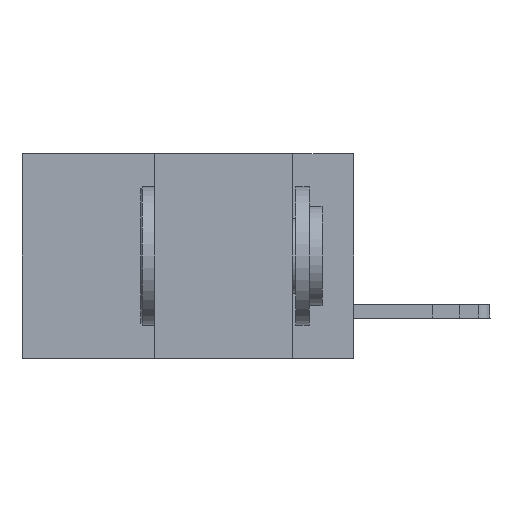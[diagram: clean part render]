
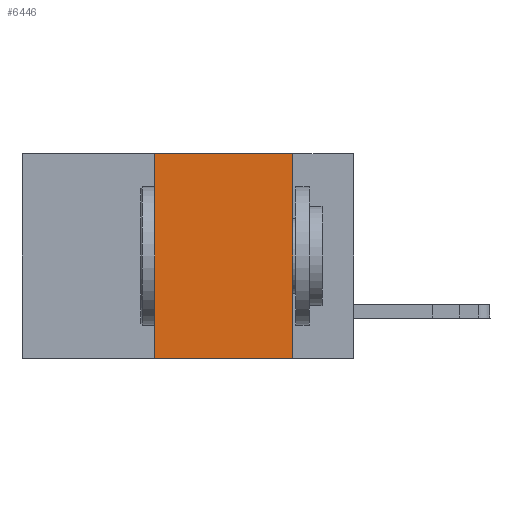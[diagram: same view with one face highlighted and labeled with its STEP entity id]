
A CAD part, left-side view. The second image highlights one B-rep face of the part: STEP entity #6446.
In plain terms, the highlighted planar face has unit normal (-1, 0, 0).
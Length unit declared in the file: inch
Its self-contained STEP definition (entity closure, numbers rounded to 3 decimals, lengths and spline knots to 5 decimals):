
#404 = LINE ( 'NONE', #10744, #22834 ) ;
#2737 = EDGE_CURVE ( 'NONE', #16615, #4697, #3067, .T. ) ;
#3067 = LINE ( 'NONE', #9073, #10866 ) ;
#4490 = PLANE ( 'NONE',  #12348 ) ;
#4584 = ORIENTED_EDGE ( 'NONE', *, *, #37653, .F. ) ;
#4697 = VERTEX_POINT ( 'NONE', #30077 ) ;
#6210 = LINE ( 'NONE', #21986, #13987 ) ;
#6305 = CARTESIAN_POINT ( 'NONE',  ( 0., 0.11, 0. ) ) ;
#6446 = ADVANCED_FACE ( 'NONE', ( #10948 ), #4490, .F. ) ;
#6537 = EDGE_CURVE ( 'NONE', #23787, #15806, #404, .T. ) ;
#7437 = DIRECTION ( 'NONE',  ( 1., 0., 0. ) ) ;
#8986 = EDGE_CURVE ( 'NONE', #15806, #4697, #12177, .T. ) ;
#9073 = CARTESIAN_POINT ( 'NONE',  ( 0., 0.6, -0.37 ) ) ;
#10744 = CARTESIAN_POINT ( 'NONE',  ( 0., 0.6, 0. ) ) ;
#10866 = VECTOR ( 'NONE', #23645, 39.37008 ) ;
#10948 = FACE_OUTER_BOUND ( 'NONE', #24705, .T. ) ;
#11093 = CARTESIAN_POINT ( 'NONE',  ( 0., 0.36, 0. ) ) ;
#12177 = LINE ( 'NONE', #16895, #26832 ) ;
#12348 = AXIS2_PLACEMENT_3D ( 'NONE', #24965, #7437, #27908 ) ;
#13987 = VECTOR ( 'NONE', #36530, 39.37008 ) ;
#14193 = ORIENTED_EDGE ( 'NONE', *, *, #2737, .T. ) ;
#15806 = VERTEX_POINT ( 'NONE', #6305 ) ;
#16615 = VERTEX_POINT ( 'NONE', #30578 ) ;
#16895 = CARTESIAN_POINT ( 'NONE',  ( 0., 0.11, 0. ) ) ;
#21986 = CARTESIAN_POINT ( 'NONE',  ( 0., 0.36, 0. ) ) ;
#22834 = VECTOR ( 'NONE', #25333, 39.37008 ) ;
#23645 = DIRECTION ( 'NONE',  ( 0., -1., 0. ) ) ;
#23787 = VERTEX_POINT ( 'NONE', #11093 ) ;
#24705 = EDGE_LOOP ( 'NONE', ( #35666, #25635, #4584, #14193 ) ) ;
#24965 = CARTESIAN_POINT ( 'NONE',  ( 0., 0.6, 0. ) ) ;
#25333 = DIRECTION ( 'NONE',  ( 0., -1., 0. ) ) ;
#25635 = ORIENTED_EDGE ( 'NONE', *, *, #6537, .F. ) ;
#25704 = DIRECTION ( 'NONE',  ( 0., 0., -1. ) ) ;
#26832 = VECTOR ( 'NONE', #25704, 39.37008 ) ;
#27908 = DIRECTION ( 'NONE',  ( 0., 0., -1. ) ) ;
#30077 = CARTESIAN_POINT ( 'NONE',  ( 0., 0.11, -0.37 ) ) ;
#30578 = CARTESIAN_POINT ( 'NONE',  ( 0., 0.36, -0.37 ) ) ;
#35666 = ORIENTED_EDGE ( 'NONE', *, *, #8986, .F. ) ;
#36530 = DIRECTION ( 'NONE',  ( 0., 0., 1. ) ) ;
#37653 = EDGE_CURVE ( 'NONE', #16615, #23787, #6210, .T. ) ;
